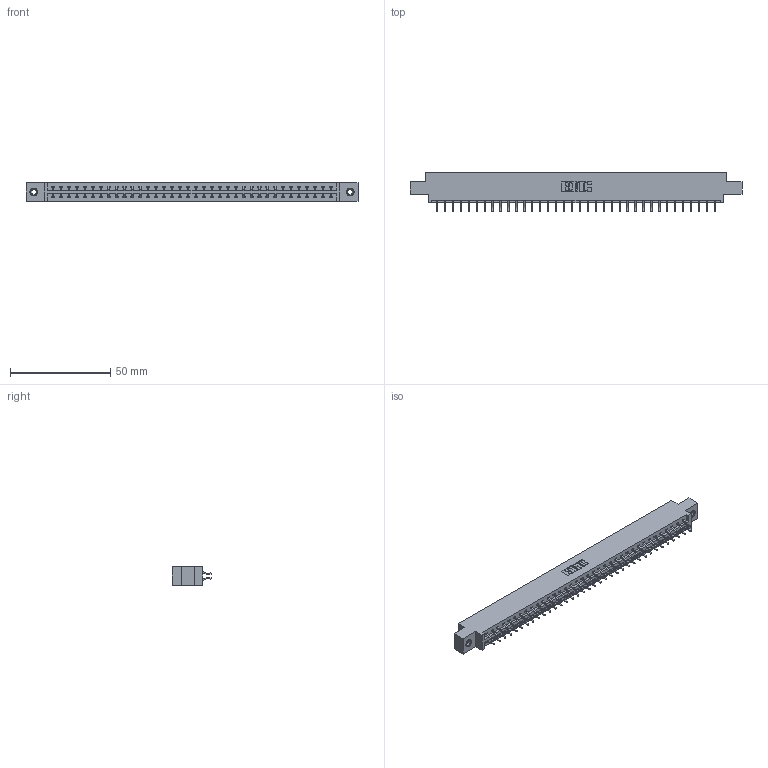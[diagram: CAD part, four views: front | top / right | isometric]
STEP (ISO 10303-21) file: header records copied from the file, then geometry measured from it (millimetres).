
FILE_DESCRIPTION (( 'STEP AP203' ), '1' );
FILE_NAME ('337-072-556-808.STEP', '2018-08-11T15:36:28', ( '' ), ( '' ), 'SwSTEP 2.0', 'SolidWorks 2016', '' );
FILE_SCHEMA (( 'CONFIG_CONTROL_DESIGN' ));
Length unit declared in the file: inch
Products named in the file (4): 345-292-001_556 Tail; 345-250-001_345-250-003-102; 337-072-556-808; 337 Part_0.170 Offset - 0.156 Dia-TI
Assembly tree (75 placements, depth 2):
  337-072-556-808
    337 Part_0.170 Offset - 0.156 Dia-TI
    345-292-001_556 Tail  x72
    345-250-001_345-250-003-102  x2
Bounding box: 165.66 x 19.57 x 9.4 mm (x, y, z)
Volume: 17251.7 mm3; surface area: 19500.6 mm2
Topology: 75 solids, 75 shells, 4498 faces, 13347 edges, 8794 vertices
Faces by surface type: plane 3130, cylinder 1352, cone 12, torus 4
Entity records: 30226 total; most frequent: CARTESIAN_POINT 5093, ORIENTED_EDGE 5010, DIRECTION 4363, EDGE_CURVE 2505, VECTOR 2349, LINE 2349, VERTEX_POINT 1664, AXIS2_PLACEMENT_3D 1007
